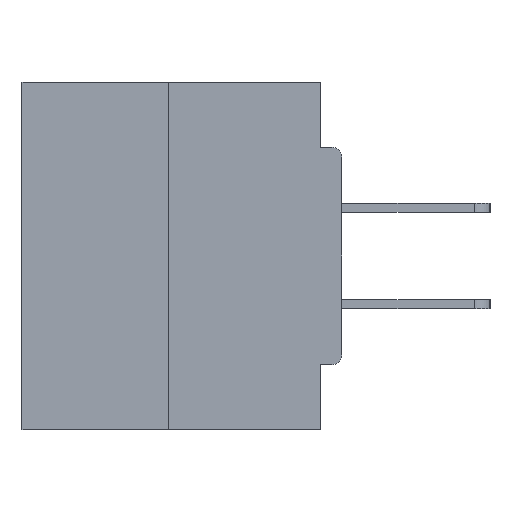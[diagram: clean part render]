
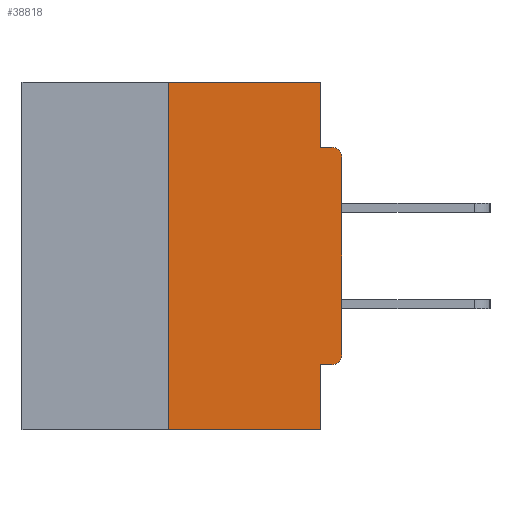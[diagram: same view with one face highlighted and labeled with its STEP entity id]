
A CAD part, left-side view. The second image highlights one B-rep face of the part: STEP entity #38818.
In plain terms, the highlighted planar face has unit normal (-1, 0, 0).
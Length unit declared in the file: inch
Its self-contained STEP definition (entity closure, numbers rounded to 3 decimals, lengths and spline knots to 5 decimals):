
#830 = VECTOR ( 'NONE', #40192, 39.37008 ) ;
#1006 = EDGE_CURVE ( 'NONE', #4723, #25486, #25771, .T. ) ;
#2037 = EDGE_CURVE ( 'NONE', #21300, #42533, #21377, .T. ) ;
#2215 = ORIENTED_EDGE ( 'NONE', *, *, #44350, .F. ) ;
#2221 = VECTOR ( 'NONE', #18882, 39.37008 ) ;
#2233 = EDGE_CURVE ( 'NONE', #4723, #42533, #41797, .T. ) ;
#2655 = CARTESIAN_POINT ( 'NONE',  ( 0., 0.031, -0.5 ) ) ;
#3978 = VECTOR ( 'NONE', #43565, 39.37008 ) ;
#4221 = DIRECTION ( 'NONE',  ( 0., 0., 1. ) ) ;
#4723 = VERTEX_POINT ( 'NONE', #21987 ) ;
#5816 = ORIENTED_EDGE ( 'NONE', *, *, #35342, .F. ) ;
#5973 = DIRECTION ( 'NONE',  ( 0., 0., -1. ) ) ;
#6043 = LINE ( 'NONE', #26636, #41601 ) ;
#6748 = VERTEX_POINT ( 'NONE', #40923 ) ;
#6839 = AXIS2_PLACEMENT_3D ( 'NONE', #13385, #9896, #5973 ) ;
#8367 = DIRECTION ( 'NONE',  ( 0., 0., -1. ) ) ;
#8920 = VERTEX_POINT ( 'NONE', #43570 ) ;
#9621 = DIRECTION ( 'NONE',  ( 0., 0., -1. ) ) ;
#9896 = DIRECTION ( 'NONE',  ( -1., 0., 0. ) ) ;
#11638 = ORIENTED_EDGE ( 'NONE', *, *, #2233, .T. ) ;
#12802 = DIRECTION ( 'NONE',  ( 0., 0., 1. ) ) ;
#13385 = CARTESIAN_POINT ( 'NONE',  ( 0., 0.015, -0.3915 ) ) ;
#13615 = VERTEX_POINT ( 'NONE', #21642 ) ;
#14742 = CARTESIAN_POINT ( 'NONE',  ( 0., 0.46, 0. ) ) ;
#15263 = CARTESIAN_POINT ( 'NONE',  ( 0., 0.031, 0. ) ) ;
#15310 = CARTESIAN_POINT ( 'NONE',  ( 0., 0.031, 0. ) ) ;
#15430 = ORIENTED_EDGE ( 'NONE', *, *, #20719, .F. ) ;
#16698 = CARTESIAN_POINT ( 'NONE',  ( 0., 0.031, -0.5 ) ) ;
#17191 = FACE_OUTER_BOUND ( 'NONE', #17437, .T. ) ;
#17437 = EDGE_LOOP ( 'NONE', ( #15430, #41153, #11638, #27130, #5816, #23830, #43964, #29818, #38171, #2215 ) ) ;
#18882 = DIRECTION ( 'NONE',  ( 0., -1., 0. ) ) ;
#20511 = CARTESIAN_POINT ( 'NONE',  ( 0., 0.015, -0.0935 ) ) ;
#20719 = EDGE_CURVE ( 'NONE', #25486, #23147, #39062, .T. ) ;
#21088 = DIRECTION ( 'NONE',  ( 0., -1., 0. ) ) ;
#21300 = VERTEX_POINT ( 'NONE', #22309 ) ;
#21377 = LINE ( 'NONE', #2655, #27277 ) ;
#21642 = CARTESIAN_POINT ( 'NONE',  ( 0., 0.031, -0.0935 ) ) ;
#21947 = PLANE ( 'NONE',  #32495 ) ;
#21987 = CARTESIAN_POINT ( 'NONE',  ( 0., 0.25, -0.5 ) ) ;
#22309 = CARTESIAN_POINT ( 'NONE',  ( 0., 0.031, -0.4065 ) ) ;
#23147 = VERTEX_POINT ( 'NONE', #15310 ) ;
#23830 = ORIENTED_EDGE ( 'NONE', *, *, #42508, .T. ) ;
#24431 = VECTOR ( 'NONE', #29220, 39.37008 ) ;
#25059 = LINE ( 'NONE', #26274, #3978 ) ;
#25196 = CIRCLE ( 'NONE', #25888, 0.015 ) ;
#25486 = VERTEX_POINT ( 'NONE', #43959 ) ;
#25564 = DIRECTION ( 'NONE',  ( 1., 0., 0. ) ) ;
#25771 = LINE ( 'NONE', #28617, #31650 ) ;
#25888 = AXIS2_PLACEMENT_3D ( 'NONE', #34647, #27902, #31321 ) ;
#26274 = CARTESIAN_POINT ( 'NONE',  ( 0., 0., -0.4065 ) ) ;
#26520 = CARTESIAN_POINT ( 'NONE',  ( 0., 0.46, 0. ) ) ;
#26636 = CARTESIAN_POINT ( 'NONE',  ( 0., 0., 0. ) ) ;
#27130 = ORIENTED_EDGE ( 'NONE', *, *, #2037, .F. ) ;
#27277 = VECTOR ( 'NONE', #9621, 39.37008 ) ;
#27902 = DIRECTION ( 'NONE',  ( -1., 0., 0. ) ) ;
#28553 = EDGE_CURVE ( 'NONE', #13615, #29526, #41044, .T. ) ;
#28617 = CARTESIAN_POINT ( 'NONE',  ( 0., 0.25, 0. ) ) ;
#29213 = EDGE_CURVE ( 'NONE', #6748, #29526, #25196, .T. ) ;
#29220 = DIRECTION ( 'NONE',  ( 0., 0., -1. ) ) ;
#29526 = VERTEX_POINT ( 'NONE', #20511 ) ;
#29818 = ORIENTED_EDGE ( 'NONE', *, *, #29213, .T. ) ;
#31321 = DIRECTION ( 'NONE',  ( 0., 0., -1. ) ) ;
#31650 = VECTOR ( 'NONE', #4221, 39.37008 ) ;
#31895 = CARTESIAN_POINT ( 'NONE',  ( 0., 0.46, -0.5 ) ) ;
#32495 = AXIS2_PLACEMENT_3D ( 'NONE', #14742, #25564, #8367 ) ;
#34647 = CARTESIAN_POINT ( 'NONE',  ( 0., 0.015, -0.1085 ) ) ;
#35342 = EDGE_CURVE ( 'NONE', #39459, #21300, #25059, .T. ) ;
#35800 = CIRCLE ( 'NONE', #6839, 0.015 ) ;
#36867 = CARTESIAN_POINT ( 'NONE',  ( 0., 0.015, -0.4065 ) ) ;
#37780 = LINE ( 'NONE', #15263, #24431 ) ;
#38171 = ORIENTED_EDGE ( 'NONE', *, *, #28553, .F. ) ;
#38818 = ADVANCED_FACE ( 'NONE', ( #17191 ), #21947, .F. ) ;
#39062 = LINE ( 'NONE', #26520, #830 ) ;
#39459 = VERTEX_POINT ( 'NONE', #36867 ) ;
#39643 = VECTOR ( 'NONE', #21088, 39.37008 ) ;
#40192 = DIRECTION ( 'NONE',  ( 0., -1., 0. ) ) ;
#40923 = CARTESIAN_POINT ( 'NONE',  ( 0., 0., -0.1085 ) ) ;
#41044 = LINE ( 'NONE', #41878, #2221 ) ;
#41153 = ORIENTED_EDGE ( 'NONE', *, *, #1006, .F. ) ;
#41601 = VECTOR ( 'NONE', #12802, 39.37008 ) ;
#41797 = LINE ( 'NONE', #31895, #39643 ) ;
#41878 = CARTESIAN_POINT ( 'NONE',  ( 0., 0., -0.0935 ) ) ;
#42508 = EDGE_CURVE ( 'NONE', #39459, #8920, #35800, .T. ) ;
#42533 = VERTEX_POINT ( 'NONE', #16698 ) ;
#43565 = DIRECTION ( 'NONE',  ( 0., 1., 0. ) ) ;
#43570 = CARTESIAN_POINT ( 'NONE',  ( 0., 0., -0.3915 ) ) ;
#43959 = CARTESIAN_POINT ( 'NONE',  ( 0., 0.25, 0. ) ) ;
#43964 = ORIENTED_EDGE ( 'NONE', *, *, #44399, .T. ) ;
#44350 = EDGE_CURVE ( 'NONE', #23147, #13615, #37780, .T. ) ;
#44399 = EDGE_CURVE ( 'NONE', #8920, #6748, #6043, .T. ) ;
